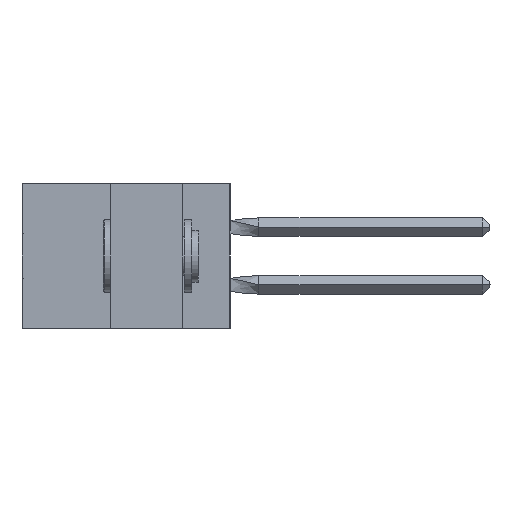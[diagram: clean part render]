
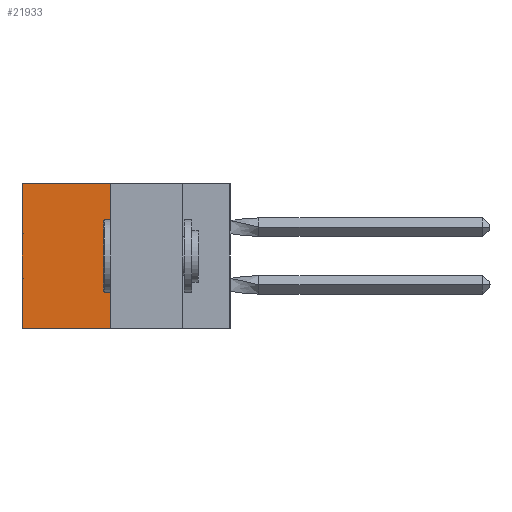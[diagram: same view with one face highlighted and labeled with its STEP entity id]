
A CAD part, left-side view. The second image highlights one B-rep face of the part: STEP entity #21933.
In plain terms, the highlighted planar face has unit normal (-1, 0, 0).
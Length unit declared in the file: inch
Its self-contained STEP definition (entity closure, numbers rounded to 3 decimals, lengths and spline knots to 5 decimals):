
#84 = VERTEX_POINT ( 'NONE', #3253 ) ;
#2146 = ORIENTED_EDGE ( 'NONE', *, *, #14070, .F. ) ;
#2239 = VECTOR ( 'NONE', #28949, 39.37008 ) ;
#2395 = ORIENTED_EDGE ( 'NONE', *, *, #4975, .T. ) ;
#3253 = CARTESIAN_POINT ( 'NONE',  ( 0.305, 0.72, -0.5 ) ) ;
#3623 = CARTESIAN_POINT ( 'NONE',  ( 0.305, 0.72, -0.5 ) ) ;
#4461 = DIRECTION ( 'NONE',  ( 0., 1., 0. ) ) ;
#4904 = EDGE_CURVE ( 'NONE', #8470, #84, #32888, .T. ) ;
#4975 = EDGE_CURVE ( 'NONE', #35616, #8470, #11633, .T. ) ;
#7443 = CARTESIAN_POINT ( 'NONE',  ( 0.305, 0.413, -0.5 ) ) ;
#8470 = VERTEX_POINT ( 'NONE', #19573 ) ;
#9313 = CARTESIAN_POINT ( 'NONE',  ( 0.305, 0.413, -0.5 ) ) ;
#11633 = LINE ( 'NONE', #44271, #28141 ) ;
#12103 = VERTEX_POINT ( 'NONE', #9313 ) ;
#13263 = ORIENTED_EDGE ( 'NONE', *, *, #4904, .T. ) ;
#14070 = EDGE_CURVE ( 'NONE', #12103, #84, #25284, .T. ) ;
#14701 = AXIS2_PLACEMENT_3D ( 'NONE', #7443, #29302, #18369 ) ;
#16773 = VECTOR ( 'NONE', #26153, 39.37008 ) ;
#18369 = DIRECTION ( 'NONE',  ( 0., 0., -1. ) ) ;
#18847 = CARTESIAN_POINT ( 'NONE',  ( 0.305, 0.413, -0.5 ) ) ;
#19573 = CARTESIAN_POINT ( 'NONE',  ( 0.305, 0.72, 0. ) ) ;
#20265 = EDGE_CURVE ( 'NONE', #35616, #12103, #28674, .T. ) ;
#21933 = ADVANCED_FACE ( 'NONE', ( #41048 ), #29133, .F. ) ;
#25284 = LINE ( 'NONE', #41275, #16773 ) ;
#26153 = DIRECTION ( 'NONE',  ( 0., 1., 0. ) ) ;
#26980 = VECTOR ( 'NONE', #29795, 39.37008 ) ;
#28141 = VECTOR ( 'NONE', #4461, 39.37008 ) ;
#28674 = LINE ( 'NONE', #18847, #26980 ) ;
#28949 = DIRECTION ( 'NONE',  ( 0., 0., -1. ) ) ;
#29133 = PLANE ( 'NONE',  #14701 ) ;
#29302 = DIRECTION ( 'NONE',  ( 1., 0., 0. ) ) ;
#29795 = DIRECTION ( 'NONE',  ( 0., 0., -1. ) ) ;
#32888 = LINE ( 'NONE', #3623, #2239 ) ;
#35616 = VERTEX_POINT ( 'NONE', #46772 ) ;
#41048 = FACE_OUTER_BOUND ( 'NONE', #41801, .T. ) ;
#41275 = CARTESIAN_POINT ( 'NONE',  ( 0.305, 0.413, -0.5 ) ) ;
#41801 = EDGE_LOOP ( 'NONE', ( #13263, #2146, #46102, #2395 ) ) ;
#44271 = CARTESIAN_POINT ( 'NONE',  ( 0.305, 0.413, 0. ) ) ;
#46102 = ORIENTED_EDGE ( 'NONE', *, *, #20265, .F. ) ;
#46772 = CARTESIAN_POINT ( 'NONE',  ( 0.305, 0.413, 0. ) ) ;
